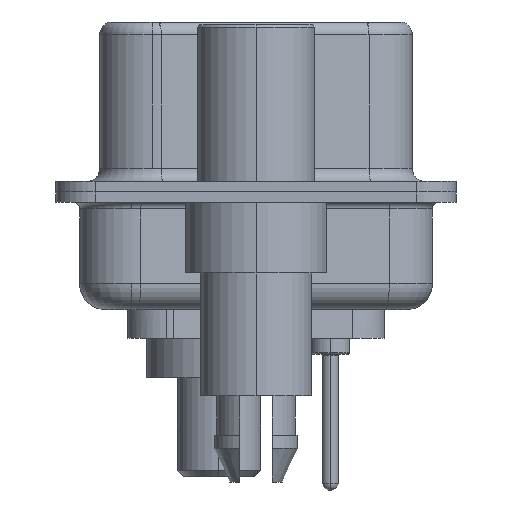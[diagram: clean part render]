
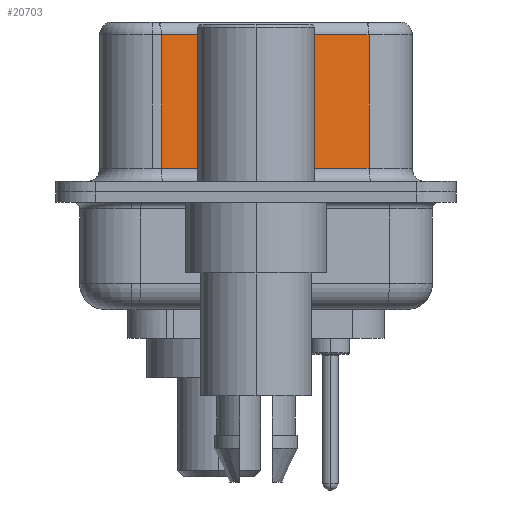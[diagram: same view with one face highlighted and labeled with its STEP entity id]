
A CAD part, left-side view. The second image highlights one B-rep face of the part: STEP entity #20703.
In plain terms, the highlighted planar face has unit normal (-0.985, -0.174, 0).
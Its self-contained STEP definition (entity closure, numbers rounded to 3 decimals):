
#27 = CARTESIAN_POINT ( 'NONE',  ( 3.73, 3.628, 6.52 ) ) ;
#191 = VERTEX_POINT ( 'NONE', #13367 ) ;
#2333 = EDGE_CURVE ( 'NONE', #191, #9823, #21126, .T. ) ;
#3325 = LINE ( 'NONE', #27, #23047 ) ;
#4471 = CARTESIAN_POINT ( 'NONE',  ( 5.132, -4.322, 6.02 ) ) ;
#4809 = VECTOR ( 'NONE', #23579, 1000. ) ;
#4993 = EDGE_LOOP ( 'NONE', ( #14605, #7157, #18851, #21888 ) ) ;
#7157 = ORIENTED_EDGE ( 'NONE', *, *, #16673, .T. ) ;
#7618 = DIRECTION ( 'NONE',  ( 0., 0., -1. ) ) ;
#7726 = DIRECTION ( 'NONE',  ( 0., 0., -1. ) ) ;
#8074 = DIRECTION ( 'NONE',  ( -0.174, 0.985, 0. ) ) ;
#8439 = EDGE_CURVE ( 'NONE', #24521, #9823, #23389, .T. ) ;
#9823 = VERTEX_POINT ( 'NONE', #20182 ) ;
#9869 = LINE ( 'NONE', #4471, #4809 ) ;
#11817 = PLANE ( 'NONE',  #13112 ) ;
#12032 = CARTESIAN_POINT ( 'NONE',  ( 5.132, -4.322, 0.9 ) ) ;
#12519 = CARTESIAN_POINT ( 'NONE',  ( 3.73, 3.628, 6.02 ) ) ;
#13112 = AXIS2_PLACEMENT_3D ( 'NONE', #23275, #19534, #8074 ) ;
#13367 = CARTESIAN_POINT ( 'NONE',  ( 5.132, -4.322, 6.02 ) ) ;
#13979 = DIRECTION ( 'NONE',  ( 0.174, -0.985, 0. ) ) ;
#14605 = ORIENTED_EDGE ( 'NONE', *, *, #2333, .F. ) ;
#16039 = VECTOR ( 'NONE', #7618, 1000. ) ;
#16486 = EDGE_CURVE ( 'NONE', #20249, #24521, #3325, .T. ) ;
#16673 = EDGE_CURVE ( 'NONE', #191, #20249, #9869, .T. ) ;
#18332 = CARTESIAN_POINT ( 'NONE',  ( 3.73, 3.628, 0.9 ) ) ;
#18851 = ORIENTED_EDGE ( 'NONE', *, *, #16486, .T. ) ;
#19534 = DIRECTION ( 'NONE',  ( 0.985, 0.174, 0. ) ) ;
#19980 = CARTESIAN_POINT ( 'NONE',  ( 5.132, -4.322, 6.52 ) ) ;
#20182 = CARTESIAN_POINT ( 'NONE',  ( 5.132, -4.322, 0.9 ) ) ;
#20249 = VERTEX_POINT ( 'NONE', #12519 ) ;
#20703 = ADVANCED_FACE ( 'NONE', ( #24681 ), #11817, .F. ) ;
#21126 = LINE ( 'NONE', #19980, #16039 ) ;
#21888 = ORIENTED_EDGE ( 'NONE', *, *, #8439, .T. ) ;
#22787 = VECTOR ( 'NONE', #13979, 1000. ) ;
#23047 = VECTOR ( 'NONE', #7726, 1000. ) ;
#23275 = CARTESIAN_POINT ( 'NONE',  ( 5.132, -4.322, 6.52 ) ) ;
#23389 = LINE ( 'NONE', #12032, #22787 ) ;
#23579 = DIRECTION ( 'NONE',  ( -0.174, 0.985, 0. ) ) ;
#24521 = VERTEX_POINT ( 'NONE', #18332 ) ;
#24681 = FACE_OUTER_BOUND ( 'NONE', #4993, .T. ) ;
